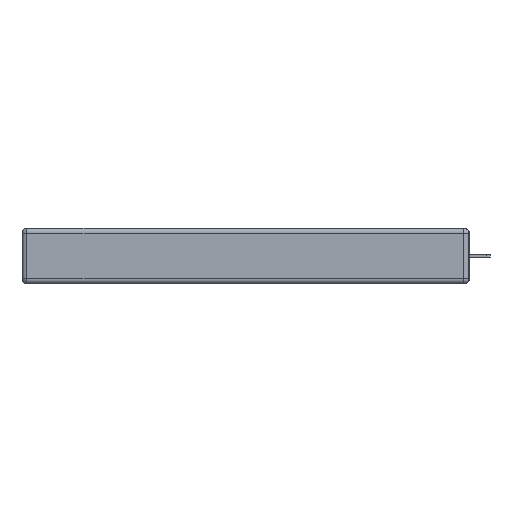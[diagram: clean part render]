
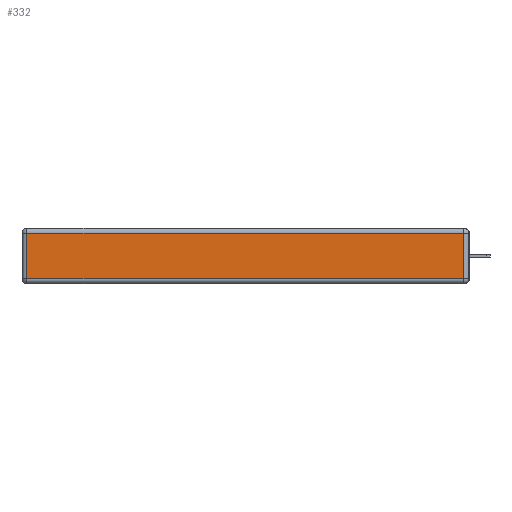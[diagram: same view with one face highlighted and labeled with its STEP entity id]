
A CAD part, left-side view. The second image highlights one B-rep face of the part: STEP entity #332.
In plain terms, the highlighted planar face has unit normal (-1, 0, 0).
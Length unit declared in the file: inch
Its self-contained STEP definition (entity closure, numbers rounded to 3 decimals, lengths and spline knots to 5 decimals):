
#332 = ADVANCED_FACE ( 'NONE', ( #16813 ), #10566, .T. ) ;
#635 = CARTESIAN_POINT ( 'NONE',  ( 0., 0.03, -0.03 ) ) ;
#1183 = ORIENTED_EDGE ( 'NONE', *, *, #7328, .T. ) ;
#1297 = DIRECTION ( 'NONE',  ( 0., 0., -1. ) ) ;
#1567 = DIRECTION ( 'NONE',  ( -1., 0., 0. ) ) ;
#1725 = DIRECTION ( 'NONE',  ( 0., 0., 1. ) ) ;
#2964 = CARTESIAN_POINT ( 'NONE',  ( 0., 2.72, -0.03 ) ) ;
#4658 = LINE ( 'NONE', #6687, #9046 ) ;
#5789 = AXIS2_PLACEMENT_3D ( 'NONE', #12209, #1567, #1725 ) ;
#6687 = CARTESIAN_POINT ( 'NONE',  ( 0., 0.03, -0.343 ) ) ;
#7328 = EDGE_CURVE ( 'NONE', #21245, #10700, #4658, .T. ) ;
#7562 = VECTOR ( 'NONE', #8173, 39.37008 ) ;
#7646 = EDGE_LOOP ( 'NONE', ( #21248, #1183, #9139, #11634 ) ) ;
#8132 = DIRECTION ( 'NONE',  ( 0., 0., 1. ) ) ;
#8173 = DIRECTION ( 'NONE',  ( 0., 1., 0. ) ) ;
#8992 = LINE ( 'NONE', #9034, #19864 ) ;
#9034 = CARTESIAN_POINT ( 'NONE',  ( 0., 0., -0.313 ) ) ;
#9046 = VECTOR ( 'NONE', #8132, 39.37008 ) ;
#9139 = ORIENTED_EDGE ( 'NONE', *, *, #9746, .T. ) ;
#9418 = VERTEX_POINT ( 'NONE', #17179 ) ;
#9746 = EDGE_CURVE ( 'NONE', #10700, #19335, #18166, .T. ) ;
#10470 = CARTESIAN_POINT ( 'NONE',  ( 0., 0.03, -0.313 ) ) ;
#10566 = PLANE ( 'NONE',  #5789 ) ;
#10700 = VERTEX_POINT ( 'NONE', #635 ) ;
#11634 = ORIENTED_EDGE ( 'NONE', *, *, #21739, .T. ) ;
#12209 = CARTESIAN_POINT ( 'NONE',  ( 0., 0., -0.343 ) ) ;
#13538 = CARTESIAN_POINT ( 'NONE',  ( 0., 2.72, -0.343 ) ) ;
#16813 = FACE_OUTER_BOUND ( 'NONE', #7646, .T. ) ;
#17158 = VECTOR ( 'NONE', #1297, 39.37008 ) ;
#17179 = CARTESIAN_POINT ( 'NONE',  ( 0., 2.72, -0.313 ) ) ;
#18166 = LINE ( 'NONE', #20271, #7562 ) ;
#19335 = VERTEX_POINT ( 'NONE', #2964 ) ;
#19363 = LINE ( 'NONE', #13538, #17158 ) ;
#19864 = VECTOR ( 'NONE', #21211, 39.37008 ) ;
#20271 = CARTESIAN_POINT ( 'NONE',  ( 0., 2.75, -0.03 ) ) ;
#21211 = DIRECTION ( 'NONE',  ( 0., -1., 0. ) ) ;
#21245 = VERTEX_POINT ( 'NONE', #10470 ) ;
#21248 = ORIENTED_EDGE ( 'NONE', *, *, #22081, .T. ) ;
#21739 = EDGE_CURVE ( 'NONE', #19335, #9418, #19363, .T. ) ;
#22081 = EDGE_CURVE ( 'NONE', #9418, #21245, #8992, .T. ) ;
